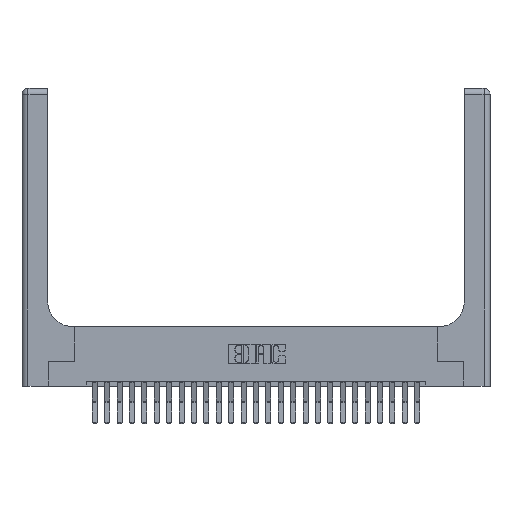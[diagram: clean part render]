
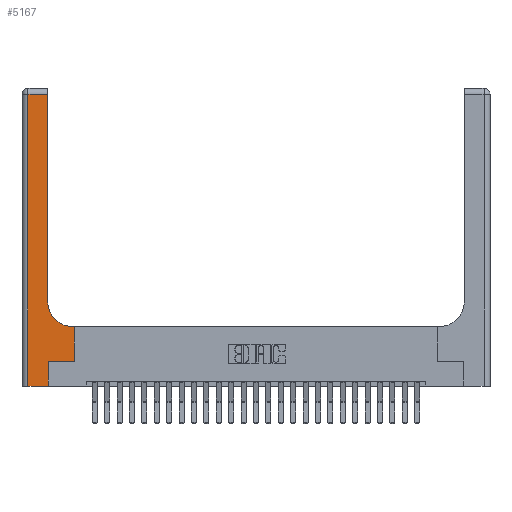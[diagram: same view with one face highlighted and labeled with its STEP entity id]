
A CAD part, top view. The second image highlights one B-rep face of the part: STEP entity #5167.
In plain terms, the highlighted planar face has unit normal (0, 0, 1).
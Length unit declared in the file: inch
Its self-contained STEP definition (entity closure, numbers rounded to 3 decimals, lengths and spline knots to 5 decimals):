
#234 = LINE ( 'NONE', #9186, #4425 ) ;
#1071 = VECTOR ( 'NONE', #19972, 39.37008 ) ;
#1080 = AXIS2_PLACEMENT_3D ( 'NONE', #16942, #3597, #18867 ) ;
#1878 = CARTESIAN_POINT ( 'NONE',  ( 0.51, 0.6, 0.37 ) ) ;
#2596 = VERTEX_POINT ( 'NONE', #1878 ) ;
#2727 = EDGE_CURVE ( 'NONE', #22834, #18491, #18459, .T. ) ;
#3311 = CARTESIAN_POINT ( 'NONE',  ( 0.51, 0.85, 0.37 ) ) ;
#3597 = DIRECTION ( 'NONE',  ( 0., 0., -1. ) ) ;
#3829 = LINE ( 'NONE', #21262, #12916 ) ;
#4183 = CARTESIAN_POINT ( 'NONE',  ( 0.528, 0.25, 0.37 ) ) ;
#4296 = EDGE_CURVE ( 'NONE', #2596, #21064, #17800, .T. ) ;
#4425 = VECTOR ( 'NONE', #24743, 39.37008 ) ;
#5118 = LINE ( 'NONE', #24445, #24119 ) ;
#5157 = ORIENTED_EDGE ( 'NONE', *, *, #18669, .T. ) ;
#5167 = ADVANCED_FACE ( 'NONE', ( #9326 ), #20734, .F. ) ;
#5221 = DIRECTION ( 'NONE',  ( 0., 0., -1. ) ) ;
#5377 = CARTESIAN_POINT ( 'NONE',  ( 0.26, 0.85, 0.37 ) ) ;
#5953 = EDGE_CURVE ( 'NONE', #19545, #2596, #6863, .T. ) ;
#6461 = CARTESIAN_POINT ( 'NONE',  ( 0.265, 0.25, 0.37 ) ) ;
#6472 = CARTESIAN_POINT ( 'NONE',  ( 0.26, 3., 0.37 ) ) ;
#6863 = LINE ( 'NONE', #10488, #17427 ) ;
#8190 = VECTOR ( 'NONE', #21655, 39.37008 ) ;
#9186 = CARTESIAN_POINT ( 'NONE',  ( 0., 0., 0.37 ) ) ;
#9326 = FACE_OUTER_BOUND ( 'NONE', #21648, .T. ) ;
#9636 = EDGE_CURVE ( 'NONE', #23780, #18754, #5118, .T. ) ;
#10132 = CARTESIAN_POINT ( 'NONE',  ( 0.528, 0.25, 0.37 ) ) ;
#10481 = ORIENTED_EDGE ( 'NONE', *, *, #9636, .T. ) ;
#10488 = CARTESIAN_POINT ( 'NONE',  ( 0.26, 0.6, 0.37 ) ) ;
#10498 = VECTOR ( 'NONE', #20033, 39.37008 ) ;
#11034 = LINE ( 'NONE', #6472, #1071 ) ;
#11675 = EDGE_CURVE ( 'NONE', #12163, #23780, #3829, .T. ) ;
#12163 = VERTEX_POINT ( 'NONE', #22915 ) ;
#12408 = ORIENTED_EDGE ( 'NONE', *, *, #11675, .T. ) ;
#12453 = ORIENTED_EDGE ( 'NONE', *, *, #4296, .T. ) ;
#12916 = VECTOR ( 'NONE', #13290, 39.37008 ) ;
#13233 = LINE ( 'NONE', #24073, #10498 ) ;
#13290 = DIRECTION ( 'NONE',  ( -1., 0., 0. ) ) ;
#13610 = DIRECTION ( 'NONE',  ( 1., 0., 0. ) ) ;
#16608 = LINE ( 'NONE', #10132, #24730 ) ;
#16815 = CARTESIAN_POINT ( 'NONE',  ( 0.06, 2.94, 0.37 ) ) ;
#16942 = CARTESIAN_POINT ( 'NONE',  ( 0., 3., 0.37 ) ) ;
#17427 = VECTOR ( 'NONE', #22108, 39.37008 ) ;
#17800 = CIRCLE ( 'NONE', #19144, 0.25 ) ;
#18302 = ORIENTED_EDGE ( 'NONE', *, *, #5953, .T. ) ;
#18459 = LINE ( 'NONE', #6461, #8190 ) ;
#18491 = VERTEX_POINT ( 'NONE', #4183 ) ;
#18669 = EDGE_CURVE ( 'NONE', #24605, #22834, #13233, .T. ) ;
#18708 = DIRECTION ( 'NONE',  ( 0., -1., 0. ) ) ;
#18754 = VERTEX_POINT ( 'NONE', #20294 ) ;
#18867 = DIRECTION ( 'NONE',  ( -1., 0., 0. ) ) ;
#19001 = ORIENTED_EDGE ( 'NONE', *, *, #19778, .T. ) ;
#19144 = AXIS2_PLACEMENT_3D ( 'NONE', #3311, #5221, #13610 ) ;
#19533 = CARTESIAN_POINT ( 'NONE',  ( 0.528, 0.6, 0.37 ) ) ;
#19545 = VERTEX_POINT ( 'NONE', #19533 ) ;
#19778 = EDGE_CURVE ( 'NONE', #18754, #24605, #234, .T. ) ;
#19972 = DIRECTION ( 'NONE',  ( 0., 1., 0. ) ) ;
#20033 = DIRECTION ( 'NONE',  ( 0., 1., 0. ) ) ;
#20294 = CARTESIAN_POINT ( 'NONE',  ( 0.06, 0., 0.37 ) ) ;
#20734 = PLANE ( 'NONE',  #1080 ) ;
#20837 = EDGE_CURVE ( 'NONE', #18491, #19545, #16608, .T. ) ;
#21064 = VERTEX_POINT ( 'NONE', #5377 ) ;
#21168 = ORIENTED_EDGE ( 'NONE', *, *, #2727, .T. ) ;
#21262 = CARTESIAN_POINT ( 'NONE',  ( 0., 2.94, 0.37 ) ) ;
#21473 = CARTESIAN_POINT ( 'NONE',  ( 0.265, 0., 0.37 ) ) ;
#21648 = EDGE_LOOP ( 'NONE', ( #21826, #12408, #10481, #19001, #5157, #21168, #23195, #18302, #12453 ) ) ;
#21655 = DIRECTION ( 'NONE',  ( 1., 0., 0. ) ) ;
#21716 = CARTESIAN_POINT ( 'NONE',  ( 0.265, 0.25, 0.37 ) ) ;
#21826 = ORIENTED_EDGE ( 'NONE', *, *, #24220, .T. ) ;
#22108 = DIRECTION ( 'NONE',  ( -1., 0., 0. ) ) ;
#22834 = VERTEX_POINT ( 'NONE', #21716 ) ;
#22915 = CARTESIAN_POINT ( 'NONE',  ( 0.26, 2.94, 0.37 ) ) ;
#23195 = ORIENTED_EDGE ( 'NONE', *, *, #20837, .T. ) ;
#23676 = DIRECTION ( 'NONE',  ( 0., 1., 0. ) ) ;
#23780 = VERTEX_POINT ( 'NONE', #16815 ) ;
#24073 = CARTESIAN_POINT ( 'NONE',  ( 0.265, 0., 0.37 ) ) ;
#24119 = VECTOR ( 'NONE', #18708, 39.37008 ) ;
#24220 = EDGE_CURVE ( 'NONE', #21064, #12163, #11034, .T. ) ;
#24445 = CARTESIAN_POINT ( 'NONE',  ( 0.06, 3., 0.37 ) ) ;
#24605 = VERTEX_POINT ( 'NONE', #21473 ) ;
#24730 = VECTOR ( 'NONE', #23676, 39.37008 ) ;
#24743 = DIRECTION ( 'NONE',  ( 1., 0., 0. ) ) ;
